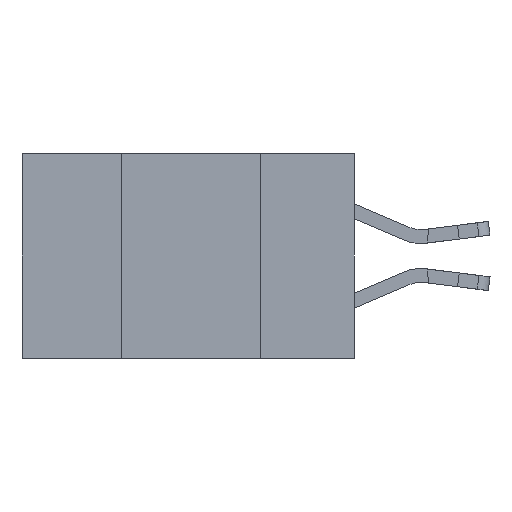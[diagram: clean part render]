
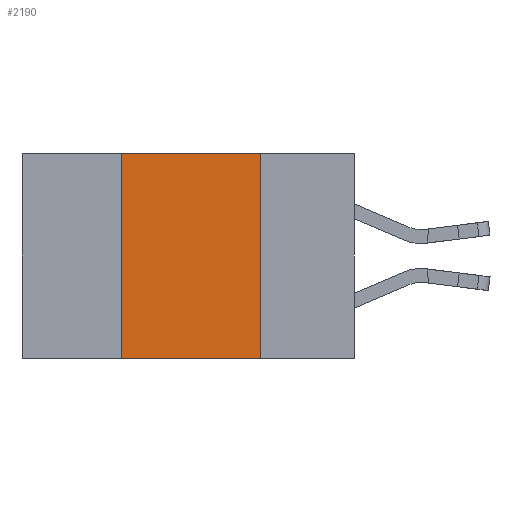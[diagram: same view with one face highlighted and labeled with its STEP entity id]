
A CAD part, left-side view. The second image highlights one B-rep face of the part: STEP entity #2190.
In plain terms, the highlighted planar face has unit normal (-1, 0, 0).
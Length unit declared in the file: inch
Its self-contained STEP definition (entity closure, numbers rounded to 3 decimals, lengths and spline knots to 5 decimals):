
#41 = ORIENTED_EDGE ( 'NONE', *, *, #4692, .F. ) ;
#542 = VECTOR ( 'NONE', #9060, 39.37008 ) ;
#567 = ORIENTED_EDGE ( 'NONE', *, *, #13019, .F. ) ;
#1387 = LINE ( 'NONE', #6400, #5119 ) ;
#1502 = EDGE_CURVE ( 'NONE', #1956, #16690, #2785, .T. ) ;
#1695 = CARTESIAN_POINT ( 'NONE',  ( 0., 0.6, 0. ) ) ;
#1854 = DIRECTION ( 'NONE',  ( 0., -1., 0. ) ) ;
#1956 = VERTEX_POINT ( 'NONE', #16512 ) ;
#2190 = ADVANCED_FACE ( 'NONE', ( #3006 ), #8172, .F. ) ;
#2785 = LINE ( 'NONE', #1695, #14736 ) ;
#3006 = FACE_OUTER_BOUND ( 'NONE', #4317, .T. ) ;
#3379 = EDGE_CURVE ( 'NONE', #15470, #17721, #19433, .T. ) ;
#4317 = EDGE_LOOP ( 'NONE', ( #41, #16158, #567, #12676 ) ) ;
#4692 = EDGE_CURVE ( 'NONE', #16690, #17721, #1387, .T. ) ;
#5119 = VECTOR ( 'NONE', #7916, 39.37008 ) ;
#5315 = CARTESIAN_POINT ( 'NONE',  ( 0., 0.42, -0.37 ) ) ;
#6400 = CARTESIAN_POINT ( 'NONE',  ( 0., 0.17, -0.37 ) ) ;
#7431 = DIRECTION ( 'NONE',  ( 0., 0., -1. ) ) ;
#7449 = DIRECTION ( 'NONE',  ( 1., 0., 0. ) ) ;
#7514 = CARTESIAN_POINT ( 'NONE',  ( 0., 0.6, 0. ) ) ;
#7781 = VECTOR ( 'NONE', #13938, 39.37008 ) ;
#7916 = DIRECTION ( 'NONE',  ( 0., 0., -1. ) ) ;
#8172 = PLANE ( 'NONE',  #17487 ) ;
#8257 = CARTESIAN_POINT ( 'NONE',  ( 0., 0.6, -0.37 ) ) ;
#9060 = DIRECTION ( 'NONE',  ( 0., 0., 1. ) ) ;
#12662 = LINE ( 'NONE', #14833, #542 ) ;
#12676 = ORIENTED_EDGE ( 'NONE', *, *, #3379, .T. ) ;
#13019 = EDGE_CURVE ( 'NONE', #15470, #1956, #12662, .T. ) ;
#13938 = DIRECTION ( 'NONE',  ( 0., -1., 0. ) ) ;
#14736 = VECTOR ( 'NONE', #1854, 39.37008 ) ;
#14833 = CARTESIAN_POINT ( 'NONE',  ( 0., 0.42, -0.37 ) ) ;
#15470 = VERTEX_POINT ( 'NONE', #5315 ) ;
#16158 = ORIENTED_EDGE ( 'NONE', *, *, #1502, .F. ) ;
#16512 = CARTESIAN_POINT ( 'NONE',  ( 0., 0.42, 0. ) ) ;
#16690 = VERTEX_POINT ( 'NONE', #18142 ) ;
#17487 = AXIS2_PLACEMENT_3D ( 'NONE', #7514, #7449, #7431 ) ;
#17721 = VERTEX_POINT ( 'NONE', #17727 ) ;
#17727 = CARTESIAN_POINT ( 'NONE',  ( 0., 0.17, -0.37 ) ) ;
#18142 = CARTESIAN_POINT ( 'NONE',  ( 0., 0.17, 0. ) ) ;
#19433 = LINE ( 'NONE', #8257, #7781 ) ;
